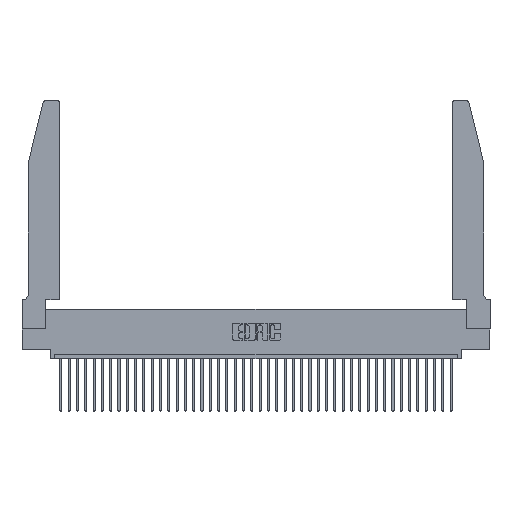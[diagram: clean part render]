
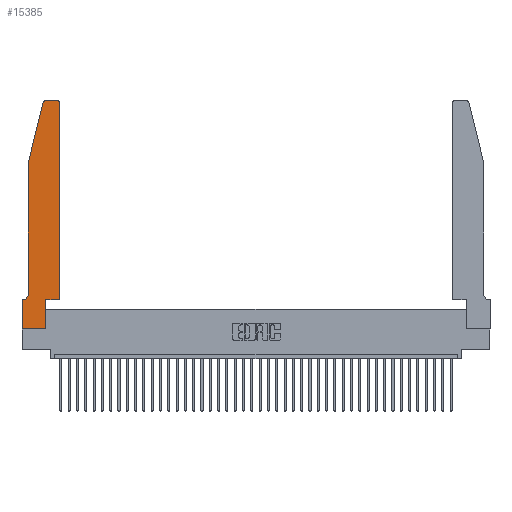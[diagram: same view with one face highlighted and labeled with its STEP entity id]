
A CAD part, top view. The second image highlights one B-rep face of the part: STEP entity #15385.
In plain terms, the highlighted planar face has unit normal (0, 0, 1).
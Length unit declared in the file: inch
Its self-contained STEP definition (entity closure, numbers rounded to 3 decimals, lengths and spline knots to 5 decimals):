
#52 = VERTEX_POINT ( 'NONE', #23768 ) ;
#829 = DIRECTION ( 'NONE',  ( 1., 0., 0. ) ) ;
#1249 = PLANE ( 'NONE',  #10394 ) ;
#1900 = VERTEX_POINT ( 'NONE', #33887 ) ;
#2087 = CARTESIAN_POINT ( 'NONE',  ( 0., 0.35, 0.37 ) ) ;
#2114 = DIRECTION ( 'NONE',  ( -1., 0., 0. ) ) ;
#2243 = VECTOR ( 'NONE', #7500, 39.37008 ) ;
#2345 = AXIS2_PLACEMENT_3D ( 'NONE', #35663, #23568, #16952 ) ;
#2409 = DIRECTION ( 'NONE',  ( 1., 0., 0. ) ) ;
#2711 = LINE ( 'NONE', #16707, #2243 ) ;
#3132 = VERTEX_POINT ( 'NONE', #2087 ) ;
#3262 = EDGE_CURVE ( 'NONE', #3132, #20487, #23895, .T. ) ;
#3631 = AXIS2_PLACEMENT_3D ( 'NONE', #38625, #5114, #2409 ) ;
#4334 = EDGE_CURVE ( 'NONE', #7582, #24772, #11913, .T. ) ;
#4520 = ORIENTED_EDGE ( 'NONE', *, *, #9393, .T. ) ;
#5052 = LINE ( 'NONE', #11743, #23475 ) ;
#5114 = DIRECTION ( 'NONE',  ( 0., 0., 1. ) ) ;
#5236 = EDGE_CURVE ( 'NONE', #24772, #10025, #5052, .T. ) ;
#5345 = CIRCLE ( 'NONE', #32765, 0.07 ) ;
#6049 = ORIENTED_EDGE ( 'NONE', *, *, #36726, .T. ) ;
#6221 = VECTOR ( 'NONE', #8851, 39.37008 ) ;
#6271 = ORIENTED_EDGE ( 'NONE', *, *, #9604, .T. ) ;
#6624 = LINE ( 'NONE', #38240, #21186 ) ;
#7500 = DIRECTION ( 'NONE',  ( 0., 1., 0. ) ) ;
#7582 = VERTEX_POINT ( 'NONE', #12082 ) ;
#8345 = DIRECTION ( 'NONE',  ( 0., 0., -1. ) ) ;
#8548 = CARTESIAN_POINT ( 'NONE',  ( 0.0755, 2., 0.37 ) ) ;
#8715 = CARTESIAN_POINT ( 'NONE',  ( 0.4505, 2.72, 0.37 ) ) ;
#8851 = DIRECTION ( 'NONE',  ( 0., 1., 0. ) ) ;
#9393 = EDGE_CURVE ( 'NONE', #15000, #37758, #37198, .T. ) ;
#9604 = EDGE_CURVE ( 'NONE', #1900, #15000, #2711, .T. ) ;
#10025 = VERTEX_POINT ( 'NONE', #32784 ) ;
#10096 = ORIENTED_EDGE ( 'NONE', *, *, #5236, .T. ) ;
#10394 = AXIS2_PLACEMENT_3D ( 'NONE', #16290, #10455, #829 ) ;
#10455 = DIRECTION ( 'NONE',  ( 0., 0., 1. ) ) ;
#10635 = ORIENTED_EDGE ( 'NONE', *, *, #4334, .T. ) ;
#11362 = CARTESIAN_POINT ( 'NONE',  ( 0.4505, 0.35, 0.37 ) ) ;
#11743 = CARTESIAN_POINT ( 'NONE',  ( 0.0755, 2., 0.37 ) ) ;
#11913 = LINE ( 'NONE', #8548, #20112 ) ;
#12082 = CARTESIAN_POINT ( 'NONE',  ( 0.25487, 2.72718, 0.37 ) ) ;
#12277 = DIRECTION ( 'NONE',  ( 0., -1., 0. ) ) ;
#12765 = EDGE_CURVE ( 'NONE', #52, #29837, #35137, .T. ) ;
#14651 = DIRECTION ( 'NONE',  ( -0.239, -0.971, 0. ) ) ;
#15000 = VERTEX_POINT ( 'NONE', #19780 ) ;
#15222 = VECTOR ( 'NONE', #38012, 39.37008 ) ;
#15304 = ORIENTED_EDGE ( 'NONE', *, *, #35502, .T. ) ;
#15378 = DIRECTION ( 'NONE',  ( -1., 0., 0. ) ) ;
#15385 = ADVANCED_FACE ( 'NONE', ( #17031 ), #1249, .T. ) ;
#15848 = ORIENTED_EDGE ( 'NONE', *, *, #25681, .T. ) ;
#15967 = EDGE_CURVE ( 'NONE', #29837, #7582, #30425, .T. ) ;
#16290 = CARTESIAN_POINT ( 'NONE',  ( 0., 0.35, 0.37 ) ) ;
#16707 = CARTESIAN_POINT ( 'NONE',  ( 0.2865, 0.35, 0.37 ) ) ;
#16952 = DIRECTION ( 'NONE',  ( 1., 0., 0. ) ) ;
#17031 = FACE_OUTER_BOUND ( 'NONE', #23423, .T. ) ;
#17450 = ORIENTED_EDGE ( 'NONE', *, *, #21564, .T. ) ;
#17729 = CIRCLE ( 'NONE', #2345, 0.03 ) ;
#18538 = ORIENTED_EDGE ( 'NONE', *, *, #15967, .T. ) ;
#18694 = DIRECTION ( 'NONE',  ( 0., -1., 0. ) ) ;
#19780 = CARTESIAN_POINT ( 'NONE',  ( 0.2865, 0.35, 0.37 ) ) ;
#19900 = CARTESIAN_POINT ( 'NONE',  ( 0.0755, 2., 0.37 ) ) ;
#20112 = VECTOR ( 'NONE', #14651, 39.37008 ) ;
#20487 = VERTEX_POINT ( 'NONE', #38844 ) ;
#20520 = LINE ( 'NONE', #28623, #15222 ) ;
#21186 = VECTOR ( 'NONE', #32375, 39.37008 ) ;
#21330 = CARTESIAN_POINT ( 'NONE',  ( 0.2605, 2.75, 0.37 ) ) ;
#21564 = EDGE_CURVE ( 'NONE', #37758, #38864, #25574, .T. ) ;
#23423 = EDGE_LOOP ( 'NONE', ( #29829, #18538, #10635, #10096, #32240, #15304, #26908, #15848, #6271, #4520, #17450, #6049 ) ) ;
#23475 = VECTOR ( 'NONE', #12277, 39.37008 ) ;
#23568 = DIRECTION ( 'NONE',  ( 0., 0., 1. ) ) ;
#23768 = CARTESIAN_POINT ( 'NONE',  ( 0.4205, 2.75, 0.37 ) ) ;
#23895 = LINE ( 'NONE', #37265, #25791 ) ;
#24772 = VERTEX_POINT ( 'NONE', #19900 ) ;
#25294 = CARTESIAN_POINT ( 'NONE',  ( 0.0055, 0.35, 0.37 ) ) ;
#25574 = LINE ( 'NONE', #36767, #6221 ) ;
#25681 = EDGE_CURVE ( 'NONE', #20487, #1900, #20520, .T. ) ;
#25791 = VECTOR ( 'NONE', #18694, 39.37008 ) ;
#26831 = VERTEX_POINT ( 'NONE', #25294 ) ;
#26908 = ORIENTED_EDGE ( 'NONE', *, *, #3262, .T. ) ;
#28528 = CARTESIAN_POINT ( 'NONE',  ( 0.4505, 0.35, 0.37 ) ) ;
#28623 = CARTESIAN_POINT ( 'NONE',  ( 0., 0., 0.37 ) ) ;
#28890 = VECTOR ( 'NONE', #33025, 39.37008 ) ;
#29829 = ORIENTED_EDGE ( 'NONE', *, *, #12765, .T. ) ;
#29837 = VERTEX_POINT ( 'NONE', #35082 ) ;
#30425 = CIRCLE ( 'NONE', #3631, 0.03 ) ;
#32240 = ORIENTED_EDGE ( 'NONE', *, *, #40056, .T. ) ;
#32375 = DIRECTION ( 'NONE',  ( -1., 0., 0. ) ) ;
#32765 = AXIS2_PLACEMENT_3D ( 'NONE', #33135, #8345, #2114 ) ;
#32784 = CARTESIAN_POINT ( 'NONE',  ( 0.0755, 0.42, 0.37 ) ) ;
#33025 = DIRECTION ( 'NONE',  ( 1., 0., 0. ) ) ;
#33135 = CARTESIAN_POINT ( 'NONE',  ( 0.0055, 0.42, 0.37 ) ) ;
#33738 = VECTOR ( 'NONE', #15378, 39.37008 ) ;
#33887 = CARTESIAN_POINT ( 'NONE',  ( 0.2865, 0., 0.37 ) ) ;
#35082 = CARTESIAN_POINT ( 'NONE',  ( 0.284, 2.75, 0.37 ) ) ;
#35137 = LINE ( 'NONE', #21330, #33738 ) ;
#35502 = EDGE_CURVE ( 'NONE', #26831, #3132, #6624, .T. ) ;
#35663 = CARTESIAN_POINT ( 'NONE',  ( 0.4205, 2.72, 0.37 ) ) ;
#36726 = EDGE_CURVE ( 'NONE', #38864, #52, #17729, .T. ) ;
#36767 = CARTESIAN_POINT ( 'NONE',  ( 0.4505, 0.35, 0.37 ) ) ;
#37198 = LINE ( 'NONE', #11362, #28890 ) ;
#37265 = CARTESIAN_POINT ( 'NONE',  ( 0., 0., 0.37 ) ) ;
#37758 = VERTEX_POINT ( 'NONE', #28528 ) ;
#38012 = DIRECTION ( 'NONE',  ( 1., 0., 0. ) ) ;
#38240 = CARTESIAN_POINT ( 'NONE',  ( 0.0755, 0.35, 0.37 ) ) ;
#38625 = CARTESIAN_POINT ( 'NONE',  ( 0.284, 2.72, 0.37 ) ) ;
#38844 = CARTESIAN_POINT ( 'NONE',  ( 0., 0., 0.37 ) ) ;
#38864 = VERTEX_POINT ( 'NONE', #8715 ) ;
#40056 = EDGE_CURVE ( 'NONE', #10025, #26831, #5345, .T. ) ;
